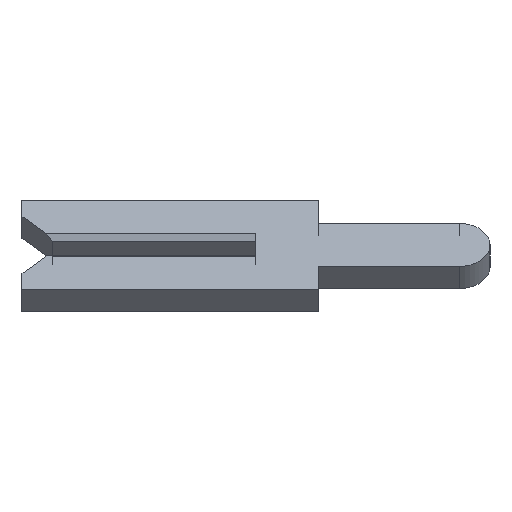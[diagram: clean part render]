
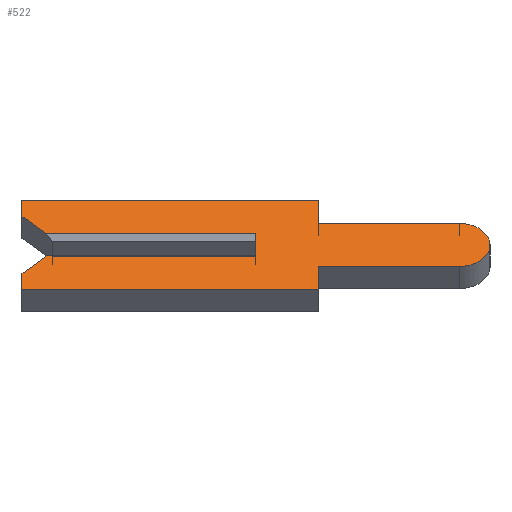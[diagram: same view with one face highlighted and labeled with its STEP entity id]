
A CAD part, left-side view. The second image highlights one B-rep face of the part: STEP entity #522.
In plain terms, the highlighted face is planar.
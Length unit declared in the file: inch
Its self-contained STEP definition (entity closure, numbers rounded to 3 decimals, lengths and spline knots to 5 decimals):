
#17 = LINE ( 'NONE', #1523, #552 ) ;
#31 = VERTEX_POINT ( 'NONE', #1660 ) ;
#32 = VECTOR ( 'NONE', #570, 39.37008 ) ;
#43 = VECTOR ( 'NONE', #536, 39.37008 ) ;
#64 = ORIENTED_EDGE ( 'NONE', *, *, #262, .F. ) ;
#100 = ORIENTED_EDGE ( 'NONE', *, *, #1182, .F. ) ;
#109 = VECTOR ( 'NONE', #1236, 39.37008 ) ;
#117 = EDGE_CURVE ( 'NONE', #2068, #581, #688, .T. ) ;
#176 = CARTESIAN_POINT ( 'NONE',  ( -0.01, -0.04, -0.0195 ) ) ;
#180 = VERTEX_POINT ( 'NONE', #1874 ) ;
#222 = EDGE_CURVE ( 'NONE', #581, #674, #848, .T. ) ;
#230 = CARTESIAN_POINT ( 'NONE',  ( -0.01, -0.04, 0.04 ) ) ;
#234 = ORIENTED_EDGE ( 'NONE', *, *, #1524, .F. ) ;
#242 = VECTOR ( 'NONE', #1500, 39.37008 ) ;
#245 = EDGE_CURVE ( 'NONE', #775, #1199, #17, .T. ) ;
#262 = EDGE_CURVE ( 'NONE', #1914, #775, #1689, .T. ) ;
#289 = AXIS2_PLACEMENT_3D ( 'NONE', #737, #2033, #412 ) ;
#297 = DIRECTION ( 'NONE',  ( 0., 0.707, 0.707 ) ) ;
#335 = ORIENTED_EDGE ( 'NONE', *, *, #531, .F. ) ;
#338 = VECTOR ( 'NONE', #1214, 39.37008 ) ;
#343 = DIRECTION ( 'NONE',  ( 0., 0., -1. ) ) ;
#346 = LINE ( 'NONE', #1003, #242 ) ;
#394 = EDGE_CURVE ( 'NONE', #427, #180, #1631, .T. ) ;
#396 = CARTESIAN_POINT ( 'NONE',  ( -0.01, 0.134, 0.01 ) ) ;
#412 = DIRECTION ( 'NONE',  ( 0., 0., -1. ) ) ;
#420 = CARTESIAN_POINT ( 'NONE',  ( -0.01, 0.15, -0.026 ) ) ;
#427 = VERTEX_POINT ( 'NONE', #396 ) ;
#441 = LINE ( 'NONE', #176, #773 ) ;
#449 = CARTESIAN_POINT ( 'NONE',  ( -0.01, 0.1305, 0.0065 ) ) ;
#484 = DIRECTION ( 'NONE',  ( 1., 0., 0. ) ) ;
#487 = VERTEX_POINT ( 'NONE', #542 ) ;
#522 = ADVANCED_FACE ( 'NONE', ( #819 ), #726, .F. ) ;
#531 = EDGE_CURVE ( 'NONE', #674, #1239, #899, .T. ) ;
#536 = DIRECTION ( 'NONE',  ( 0., 0., -1. ) ) ;
#542 = CARTESIAN_POINT ( 'NONE',  ( -0.01, 0.15, 0.04 ) ) ;
#548 = LINE ( 'NONE', #1384, #1774 ) ;
#549 = DIRECTION ( 'NONE',  ( 0., 0., 1. ) ) ;
#552 = VECTOR ( 'NONE', #564, 39.37008 ) ;
#557 = CARTESIAN_POINT ( 'NONE',  ( -0.01, 0.15, -0.04 ) ) ;
#564 = DIRECTION ( 'NONE',  ( 0., -1., 0. ) ) ;
#568 = ORIENTED_EDGE ( 'NONE', *, *, #842, .F. ) ;
#570 = DIRECTION ( 'NONE',  ( 0., -1., 0. ) ) ;
#581 = VERTEX_POINT ( 'NONE', #557 ) ;
#589 = ORIENTED_EDGE ( 'NONE', *, *, #222, .F. ) ;
#593 = LINE ( 'NONE', #449, #1503 ) ;
#599 = ORIENTED_EDGE ( 'NONE', *, *, #929, .F. ) ;
#610 = CARTESIAN_POINT ( 'NONE',  ( -0.01, 0.134, -0.01 ) ) ;
#662 = CARTESIAN_POINT ( 'NONE',  ( -0.01, 0.15, 0.04 ) ) ;
#674 = VERTEX_POINT ( 'NONE', #420 ) ;
#688 = LINE ( 'NONE', #1812, #1715 ) ;
#726 = PLANE ( 'NONE',  #289 ) ;
#737 = CARTESIAN_POINT ( 'NONE',  ( -0.01, -0.1305, 0. ) ) ;
#759 = VECTOR ( 'NONE', #2043, 39.37008 ) ;
#773 = VECTOR ( 'NONE', #1847, 39.37008 ) ;
#775 = VERTEX_POINT ( 'NONE', #1542 ) ;
#806 = CARTESIAN_POINT ( 'NONE',  ( -0.01, -0.1305, 0.0195 ) ) ;
#819 = FACE_OUTER_BOUND ( 'NONE', #1124, .T. ) ;
#842 = EDGE_CURVE ( 'NONE', #1239, #1889, #973, .T. ) ;
#848 = LINE ( 'NONE', #1504, #1664 ) ;
#857 = DIRECTION ( 'NONE',  ( 0., 1., 0. ) ) ;
#858 = VERTEX_POINT ( 'NONE', #1072 ) ;
#866 = CARTESIAN_POINT ( 'NONE',  ( -0.01, -0.04, -0.04 ) ) ;
#899 = LINE ( 'NONE', #1339, #759 ) ;
#904 = ORIENTED_EDGE ( 'NONE', *, *, #1937, .F. ) ;
#913 = ORIENTED_EDGE ( 'NONE', *, *, #394, .T. ) ;
#929 = EDGE_CURVE ( 'NONE', #858, #2068, #1053, .T. ) ;
#973 = LINE ( 'NONE', #1066, #32 ) ;
#977 = EDGE_CURVE ( 'NONE', #1889, #180, #548, .T. ) ;
#991 = DIRECTION ( 'NONE',  ( 0., -1., 0. ) ) ;
#1003 = CARTESIAN_POINT ( 'NONE',  ( -0.01, 0.15, 0.026 ) ) ;
#1053 = LINE ( 'NONE', #2061, #109 ) ;
#1066 = CARTESIAN_POINT ( 'NONE',  ( -0.01, -0.1305, -0.01 ) ) ;
#1068 = CIRCLE ( 'NONE', #1526, 0.0195 ) ;
#1072 = CARTESIAN_POINT ( 'NONE',  ( -0.01, -0.04, -0.0195 ) ) ;
#1077 = ORIENTED_EDGE ( 'NONE', *, *, #977, .F. ) ;
#1082 = ORIENTED_EDGE ( 'NONE', *, *, #245, .F. ) ;
#1124 = EDGE_LOOP ( 'NONE', ( #913, #1077, #568, #335, #589, #1742, #599, #904, #1627, #1082, #64, #234, #1616, #100 ) ) ;
#1134 = CARTESIAN_POINT ( 'NONE',  ( -0.01, -0.1305, 0. ) ) ;
#1147 = CARTESIAN_POINT ( 'NONE',  ( -0.01, 0., -0.01 ) ) ;
#1182 = EDGE_CURVE ( 'NONE', #427, #31, #593, .T. ) ;
#1199 = VERTEX_POINT ( 'NONE', #806 ) ;
#1214 = DIRECTION ( 'NONE',  ( 0., -1., 0. ) ) ;
#1218 = DIRECTION ( 'NONE',  ( 0., 0., 1. ) ) ;
#1236 = DIRECTION ( 'NONE',  ( 0., 0., -1. ) ) ;
#1239 = VERTEX_POINT ( 'NONE', #610 ) ;
#1259 = CARTESIAN_POINT ( 'NONE',  ( -0.01, -0.1305, -0.0195 ) ) ;
#1339 = CARTESIAN_POINT ( 'NONE',  ( -0.01, 0.1305, -0.0065 ) ) ;
#1342 = VERTEX_POINT ( 'NONE', #1259 ) ;
#1384 = CARTESIAN_POINT ( 'NONE',  ( -0.01, 0., 0.0065 ) ) ;
#1500 = DIRECTION ( 'NONE',  ( 0., 0., 1. ) ) ;
#1503 = VECTOR ( 'NONE', #297, 39.37008 ) ;
#1504 = CARTESIAN_POINT ( 'NONE',  ( -0.01, 0.15, -0.026 ) ) ;
#1523 = CARTESIAN_POINT ( 'NONE',  ( -0.01, -0.04, 0.0195 ) ) ;
#1524 = EDGE_CURVE ( 'NONE', #487, #1914, #2036, .T. ) ;
#1526 = AXIS2_PLACEMENT_3D ( 'NONE', #1134, #484, #343 ) ;
#1542 = CARTESIAN_POINT ( 'NONE',  ( -0.01, -0.04, 0.0195 ) ) ;
#1586 = VECTOR ( 'NONE', #991, 39.37008 ) ;
#1616 = ORIENTED_EDGE ( 'NONE', *, *, #2012, .F. ) ;
#1627 = ORIENTED_EDGE ( 'NONE', *, *, #1677, .F. ) ;
#1631 = LINE ( 'NONE', #2035, #338 ) ;
#1660 = CARTESIAN_POINT ( 'NONE',  ( -0.01, 0.15, 0.026 ) ) ;
#1664 = VECTOR ( 'NONE', #549, 39.37008 ) ;
#1677 = EDGE_CURVE ( 'NONE', #1199, #1342, #1068, .T. ) ;
#1689 = LINE ( 'NONE', #230, #43 ) ;
#1715 = VECTOR ( 'NONE', #857, 39.37008 ) ;
#1742 = ORIENTED_EDGE ( 'NONE', *, *, #117, .F. ) ;
#1774 = VECTOR ( 'NONE', #1218, 39.37008 ) ;
#1812 = CARTESIAN_POINT ( 'NONE',  ( -0.01, 0.15, -0.04 ) ) ;
#1841 = CARTESIAN_POINT ( 'NONE',  ( -0.01, -0.04, 0.04 ) ) ;
#1847 = DIRECTION ( 'NONE',  ( 0., 1., 0. ) ) ;
#1874 = CARTESIAN_POINT ( 'NONE',  ( -0.01, 0., 0.01 ) ) ;
#1889 = VERTEX_POINT ( 'NONE', #1147 ) ;
#1914 = VERTEX_POINT ( 'NONE', #1841 ) ;
#1937 = EDGE_CURVE ( 'NONE', #1342, #858, #441, .T. ) ;
#2012 = EDGE_CURVE ( 'NONE', #31, #487, #346, .T. ) ;
#2033 = DIRECTION ( 'NONE',  ( 1., 0., 0. ) ) ;
#2035 = CARTESIAN_POINT ( 'NONE',  ( -0.01, 0.15, 0.01 ) ) ;
#2036 = LINE ( 'NONE', #662, #1586 ) ;
#2043 = DIRECTION ( 'NONE',  ( 0., -0.707, 0.707 ) ) ;
#2061 = CARTESIAN_POINT ( 'NONE',  ( -0.01, -0.04, -0.04 ) ) ;
#2068 = VERTEX_POINT ( 'NONE', #866 ) ;
